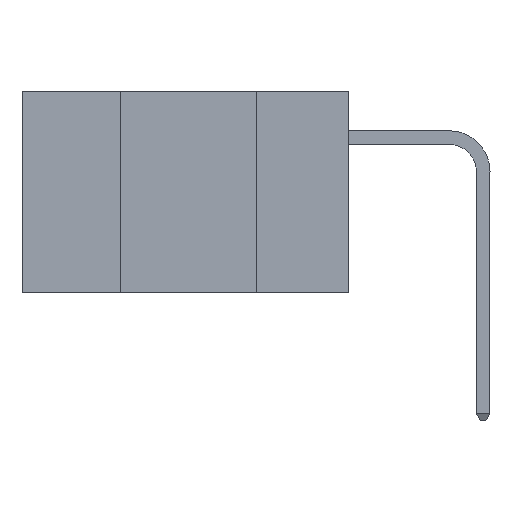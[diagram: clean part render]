
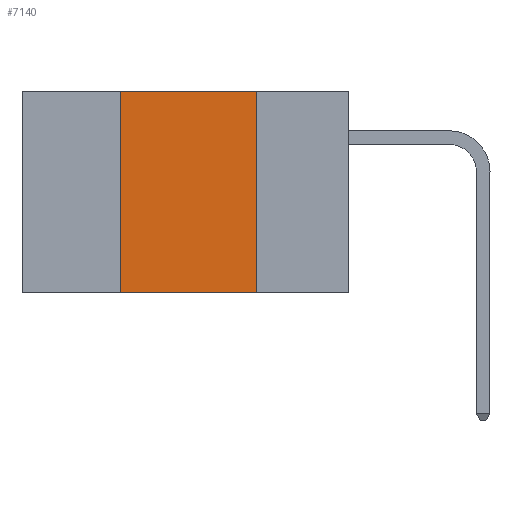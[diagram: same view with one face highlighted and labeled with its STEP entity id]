
A CAD part, left-side view. The second image highlights one B-rep face of the part: STEP entity #7140.
In plain terms, the highlighted planar face has unit normal (-1, 0, 0).
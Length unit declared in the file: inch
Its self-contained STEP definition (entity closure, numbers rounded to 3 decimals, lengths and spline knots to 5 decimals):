
#195 = CARTESIAN_POINT ( 'NONE',  ( 0., 0.17, 0. ) ) ;
#393 = DIRECTION ( 'NONE',  ( 0., 0., -1. ) ) ;
#3125 = DIRECTION ( 'NONE',  ( 1., 0., 0. ) ) ;
#3587 = LINE ( 'NONE', #11535, #16970 ) ;
#3836 = ORIENTED_EDGE ( 'NONE', *, *, #10232, .T. ) ;
#4049 = LINE ( 'NONE', #20154, #19590 ) ;
#6311 = VECTOR ( 'NONE', #393, 39.37008 ) ;
#6464 = VECTOR ( 'NONE', #17504, 39.37008 ) ;
#7140 = ADVANCED_FACE ( 'NONE', ( #24147 ), #21824, .F. ) ;
#9122 = ORIENTED_EDGE ( 'NONE', *, *, #11137, .F. ) ;
#10232 = EDGE_CURVE ( 'NONE', #25430, #14851, #4049, .T. ) ;
#11137 = EDGE_CURVE ( 'NONE', #25430, #22973, #3587, .T. ) ;
#11535 = CARTESIAN_POINT ( 'NONE',  ( 0., 0.42, 0. ) ) ;
#11844 = EDGE_LOOP ( 'NONE', ( #19293, #15516, #9122, #3836 ) ) ;
#11929 = EDGE_CURVE ( 'NONE', #22973, #14281, #18756, .T. ) ;
#13737 = CARTESIAN_POINT ( 'NONE',  ( 0., 0.17, -0.37 ) ) ;
#14281 = VERTEX_POINT ( 'NONE', #23254 ) ;
#14851 = VERTEX_POINT ( 'NONE', #13737 ) ;
#14866 = DIRECTION ( 'NONE',  ( 0., 0., -1. ) ) ;
#15516 = ORIENTED_EDGE ( 'NONE', *, *, #11929, .F. ) ;
#16562 = CARTESIAN_POINT ( 'NONE',  ( 0., 0.42, -0.37 ) ) ;
#16652 = DIRECTION ( 'NONE',  ( 0., 0., 1. ) ) ;
#16970 = VECTOR ( 'NONE', #16652, 39.37008 ) ;
#17504 = DIRECTION ( 'NONE',  ( 0., -1., 0. ) ) ;
#18756 = LINE ( 'NONE', #22041, #6464 ) ;
#18764 = EDGE_CURVE ( 'NONE', #14281, #14851, #27259, .T. ) ;
#19293 = ORIENTED_EDGE ( 'NONE', *, *, #18764, .F. ) ;
#19590 = VECTOR ( 'NONE', #24782, 39.37008 ) ;
#20154 = CARTESIAN_POINT ( 'NONE',  ( 0., 0.6, -0.37 ) ) ;
#21824 = PLANE ( 'NONE',  #27519 ) ;
#22041 = CARTESIAN_POINT ( 'NONE',  ( 0., 0.6, 0. ) ) ;
#22973 = VERTEX_POINT ( 'NONE', #24876 ) ;
#23254 = CARTESIAN_POINT ( 'NONE',  ( 0., 0.17, 0. ) ) ;
#24144 = CARTESIAN_POINT ( 'NONE',  ( 0., 0.6, 0. ) ) ;
#24147 = FACE_OUTER_BOUND ( 'NONE', #11844, .T. ) ;
#24782 = DIRECTION ( 'NONE',  ( 0., -1., 0. ) ) ;
#24876 = CARTESIAN_POINT ( 'NONE',  ( 0., 0.42, 0. ) ) ;
#25430 = VERTEX_POINT ( 'NONE', #16562 ) ;
#27259 = LINE ( 'NONE', #195, #6311 ) ;
#27519 = AXIS2_PLACEMENT_3D ( 'NONE', #24144, #3125, #14866 ) ;
